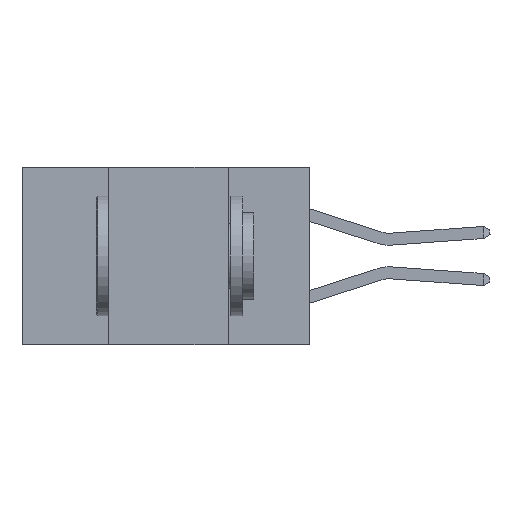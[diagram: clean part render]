
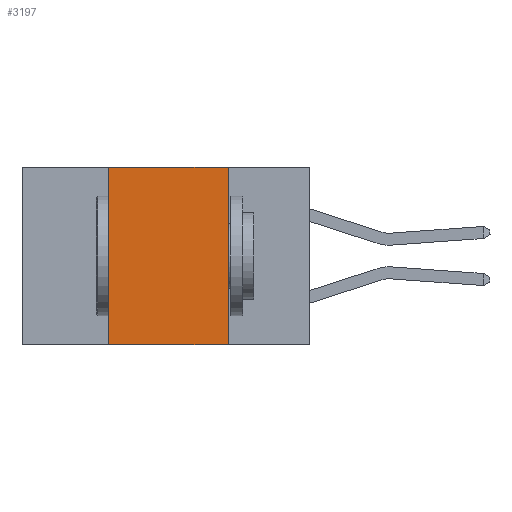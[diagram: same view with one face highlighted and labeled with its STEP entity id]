
A CAD part, left-side view. The second image highlights one B-rep face of the part: STEP entity #3197.
In plain terms, the highlighted planar face has unit normal (-1, 0, 0).
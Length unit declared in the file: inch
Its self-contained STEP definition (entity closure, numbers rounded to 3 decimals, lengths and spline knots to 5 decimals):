
#879 = LINE ( 'NONE', #5326, #8768 ) ;
#947 = ORIENTED_EDGE ( 'NONE', *, *, #4942, .F. ) ;
#990 = EDGE_CURVE ( 'NONE', #8969, #1187, #5303, .T. ) ;
#1187 = VERTEX_POINT ( 'NONE', #9227 ) ;
#1866 = CARTESIAN_POINT ( 'NONE',  ( 0., 0.6, 0. ) ) ;
#1927 = ORIENTED_EDGE ( 'NONE', *, *, #990, .T. ) ;
#1957 = ORIENTED_EDGE ( 'NONE', *, *, #7491, .F. ) ;
#2107 = AXIS2_PLACEMENT_3D ( 'NONE', #1866, #9346, #9343 ) ;
#2391 = CARTESIAN_POINT ( 'NONE',  ( 0., 0.17, -0.37 ) ) ;
#2760 = CARTESIAN_POINT ( 'NONE',  ( 0., 0.17, 0. ) ) ;
#2829 = ORIENTED_EDGE ( 'NONE', *, *, #4637, .F. ) ;
#3187 = DIRECTION ( 'NONE',  ( 0., 0., -1. ) ) ;
#3197 = ADVANCED_FACE ( 'NONE', ( #9276 ), #9382, .F. ) ;
#3423 = VECTOR ( 'NONE', #3187, 39.37008 ) ;
#4189 = CARTESIAN_POINT ( 'NONE',  ( 0., 0.6, -0.37 ) ) ;
#4637 = EDGE_CURVE ( 'NONE', #8969, #8355, #7861, .T. ) ;
#4760 = DIRECTION ( 'NONE',  ( 0., -1., 0. ) ) ;
#4942 = EDGE_CURVE ( 'NONE', #8355, #9447, #879, .T. ) ;
#5200 = CARTESIAN_POINT ( 'NONE',  ( 0., 0.42, -0.37 ) ) ;
#5303 = LINE ( 'NONE', #4189, #7088 ) ;
#5326 = CARTESIAN_POINT ( 'NONE',  ( 0., 0.6, 0. ) ) ;
#5554 = EDGE_LOOP ( 'NONE', ( #1957, #947, #2829, #1927 ) ) ;
#7088 = VECTOR ( 'NONE', #4760, 39.37008 ) ;
#7491 = EDGE_CURVE ( 'NONE', #9447, #1187, #7648, .T. ) ;
#7648 = LINE ( 'NONE', #2391, #3423 ) ;
#7840 = CARTESIAN_POINT ( 'NONE',  ( 0., 0.42, -0.37 ) ) ;
#7861 = LINE ( 'NONE', #7840, #9810 ) ;
#8243 = CARTESIAN_POINT ( 'NONE',  ( 0., 0.42, 0. ) ) ;
#8355 = VERTEX_POINT ( 'NONE', #8243 ) ;
#8768 = VECTOR ( 'NONE', #9107, 39.37008 ) ;
#8969 = VERTEX_POINT ( 'NONE', #5200 ) ;
#9107 = DIRECTION ( 'NONE',  ( 0., -1., 0. ) ) ;
#9194 = DIRECTION ( 'NONE',  ( 0., 0., 1. ) ) ;
#9227 = CARTESIAN_POINT ( 'NONE',  ( 0., 0.17, -0.37 ) ) ;
#9276 = FACE_OUTER_BOUND ( 'NONE', #5554, .T. ) ;
#9343 = DIRECTION ( 'NONE',  ( 0., 0., -1. ) ) ;
#9346 = DIRECTION ( 'NONE',  ( 1., 0., 0. ) ) ;
#9382 = PLANE ( 'NONE',  #2107 ) ;
#9447 = VERTEX_POINT ( 'NONE', #2760 ) ;
#9810 = VECTOR ( 'NONE', #9194, 39.37008 ) ;
